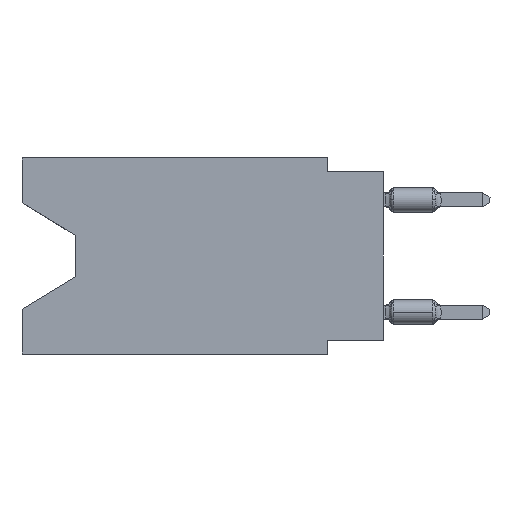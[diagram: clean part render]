
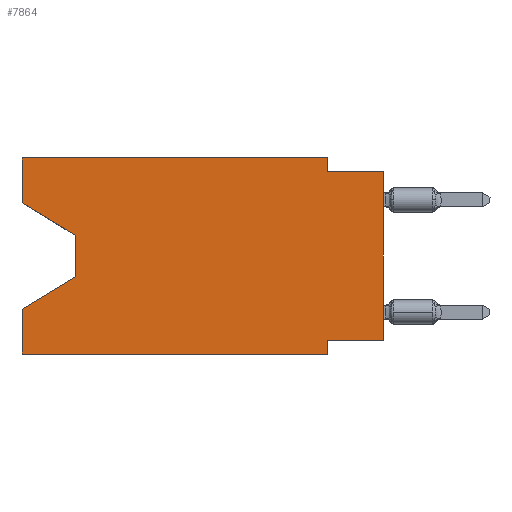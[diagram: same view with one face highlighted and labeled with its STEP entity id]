
A CAD part, left-side view. The second image highlights one B-rep face of the part: STEP entity #7864.
In plain terms, the highlighted planar face has unit normal (-1, 0, 0).
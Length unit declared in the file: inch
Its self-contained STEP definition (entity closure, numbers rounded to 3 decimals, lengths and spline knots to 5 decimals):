
#218 = ORIENTED_EDGE ( 'NONE', *, *, #9292, .T. ) ;
#283 = LINE ( 'NONE', #16107, #18698 ) ;
#565 = ORIENTED_EDGE ( 'NONE', *, *, #13233, .F. ) ;
#764 = CARTESIAN_POINT ( 'NONE',  ( 0., 0.645, -0.08025 ) ) ;
#988 = LINE ( 'NONE', #1072, #13239 ) ;
#1072 = CARTESIAN_POINT ( 'NONE',  ( 0., 0.645, 0. ) ) ;
#1233 = CARTESIAN_POINT ( 'NONE',  ( 0., 0., -0.325 ) ) ;
#1372 = EDGE_CURVE ( 'NONE', #12256, #6926, #4686, .T. ) ;
#1374 = VERTEX_POINT ( 'NONE', #11987 ) ;
#1750 = LINE ( 'NONE', #13599, #11968 ) ;
#2251 = VERTEX_POINT ( 'NONE', #5177 ) ;
#2436 = EDGE_CURVE ( 'NONE', #12759, #13123, #7107, .T. ) ;
#2453 = CARTESIAN_POINT ( 'NONE',  ( 0., 0.1, -0.35 ) ) ;
#2687 = EDGE_CURVE ( 'NONE', #2251, #11540, #3376, .T. ) ;
#3064 = ORIENTED_EDGE ( 'NONE', *, *, #10776, .F. ) ;
#3078 = ORIENTED_EDGE ( 'NONE', *, *, #2687, .F. ) ;
#3376 = LINE ( 'NONE', #6210, #5145 ) ;
#3420 = LINE ( 'NONE', #12143, #15102 ) ;
#3928 = CARTESIAN_POINT ( 'NONE',  ( 0., 0., -0.325 ) ) ;
#4103 = DIRECTION ( 'NONE',  ( 0., 0., 1. ) ) ;
#4405 = CARTESIAN_POINT ( 'NONE',  ( 0., 0.645, -0.08025 ) ) ;
#4410 = CARTESIAN_POINT ( 'NONE',  ( 0., 0.645, -0.35 ) ) ;
#4476 = LINE ( 'NONE', #10816, #8887 ) ;
#4483 = CARTESIAN_POINT ( 'NONE',  ( 0., 0.645, 0. ) ) ;
#4591 = DIRECTION ( 'NONE',  ( 0., 0., -1. ) ) ;
#4645 = DIRECTION ( 'NONE',  ( 0., 0., -1. ) ) ;
#4686 = LINE ( 'NONE', #4405, #13394 ) ;
#4913 = ORIENTED_EDGE ( 'NONE', *, *, #15853, .F. ) ;
#5021 = DIRECTION ( 'NONE',  ( 0., 0., -1. ) ) ;
#5068 = DIRECTION ( 'NONE',  ( 0., 0., 1. ) ) ;
#5093 = ORIENTED_EDGE ( 'NONE', *, *, #5103, .T. ) ;
#5103 = EDGE_CURVE ( 'NONE', #2251, #7350, #7436, .T. ) ;
#5145 = VECTOR ( 'NONE', #5068, 39.37008 ) ;
#5177 = CARTESIAN_POINT ( 'NONE',  ( 0., 0.645, -0.35 ) ) ;
#5553 = CARTESIAN_POINT ( 'NONE',  ( 0., 0.645, 0. ) ) ;
#5867 = ORIENTED_EDGE ( 'NONE', *, *, #6647, .F. ) ;
#6096 = CARTESIAN_POINT ( 'NONE',  ( 0., 0.645, 0. ) ) ;
#6210 = CARTESIAN_POINT ( 'NONE',  ( 0., 0.645, 0. ) ) ;
#6647 = EDGE_CURVE ( 'NONE', #10743, #1374, #15863, .T. ) ;
#6926 = VERTEX_POINT ( 'NONE', #7193 ) ;
#7012 = DIRECTION ( 'NONE',  ( 0., 1., 0. ) ) ;
#7064 = LINE ( 'NONE', #11426, #13480 ) ;
#7107 = LINE ( 'NONE', #1233, #17147 ) ;
#7193 = CARTESIAN_POINT ( 'NONE',  ( 0., 0.55, -0.138 ) ) ;
#7350 = VERTEX_POINT ( 'NONE', #2453 ) ;
#7428 = PLANE ( 'NONE',  #14197 ) ;
#7436 = LINE ( 'NONE', #4410, #8247 ) ;
#7521 = VECTOR ( 'NONE', #10127, 39.37008 ) ;
#7553 = CARTESIAN_POINT ( 'NONE',  ( 0., 0.55, -0.212 ) ) ;
#7864 = ADVANCED_FACE ( 'NONE', ( #16236 ), #7428, .F. ) ;
#8247 = VECTOR ( 'NONE', #13033, 39.37008 ) ;
#8756 = VERTEX_POINT ( 'NONE', #17181 ) ;
#8800 = CARTESIAN_POINT ( 'NONE',  ( 0., 0.645, -0.26975 ) ) ;
#8887 = VECTOR ( 'NONE', #5021, 39.37008 ) ;
#9042 = DIRECTION ( 'NONE',  ( 0., -0.855, -0.519 ) ) ;
#9056 = VERTEX_POINT ( 'NONE', #12149 ) ;
#9292 = EDGE_CURVE ( 'NONE', #6926, #10417, #283, .T. ) ;
#9681 = VECTOR ( 'NONE', #11416, 39.37008 ) ;
#10035 = LINE ( 'NONE', #17334, #7521 ) ;
#10127 = DIRECTION ( 'NONE',  ( 0., 0., 1. ) ) ;
#10173 = ORIENTED_EDGE ( 'NONE', *, *, #1372, .T. ) ;
#10417 = VERTEX_POINT ( 'NONE', #7553 ) ;
#10719 = ORIENTED_EDGE ( 'NONE', *, *, #2436, .F. ) ;
#10743 = VERTEX_POINT ( 'NONE', #5553 ) ;
#10776 = EDGE_CURVE ( 'NONE', #8756, #9056, #7064, .T. ) ;
#10816 = CARTESIAN_POINT ( 'NONE',  ( 0., 0.1, 0. ) ) ;
#10830 = EDGE_CURVE ( 'NONE', #10417, #11540, #1750, .T. ) ;
#11258 = EDGE_CURVE ( 'NONE', #1374, #8756, #4476, .T. ) ;
#11416 = DIRECTION ( 'NONE',  ( 0., -1., 0. ) ) ;
#11426 = CARTESIAN_POINT ( 'NONE',  ( 0., 0., -0.025 ) ) ;
#11540 = VERTEX_POINT ( 'NONE', #8800 ) ;
#11968 = VECTOR ( 'NONE', #17577, 39.37008 ) ;
#11987 = CARTESIAN_POINT ( 'NONE',  ( 0., 0.1, 0. ) ) ;
#12143 = CARTESIAN_POINT ( 'NONE',  ( 0., 0.1, -0.35 ) ) ;
#12149 = CARTESIAN_POINT ( 'NONE',  ( 0., 0., -0.025 ) ) ;
#12256 = VERTEX_POINT ( 'NONE', #764 ) ;
#12720 = ORIENTED_EDGE ( 'NONE', *, *, #14883, .T. ) ;
#12759 = VERTEX_POINT ( 'NONE', #3928 ) ;
#13033 = DIRECTION ( 'NONE',  ( 0., -1., 0. ) ) ;
#13123 = VERTEX_POINT ( 'NONE', #14909 ) ;
#13233 = EDGE_CURVE ( 'NONE', #12256, #10743, #988, .T. ) ;
#13239 = VECTOR ( 'NONE', #4103, 39.37008 ) ;
#13394 = VECTOR ( 'NONE', #9042, 39.37008 ) ;
#13480 = VECTOR ( 'NONE', #14166, 39.37008 ) ;
#13599 = CARTESIAN_POINT ( 'NONE',  ( 0., 0.55, -0.212 ) ) ;
#14166 = DIRECTION ( 'NONE',  ( 0., -1., 0. ) ) ;
#14197 = AXIS2_PLACEMENT_3D ( 'NONE', #6096, #14344, #4591 ) ;
#14344 = DIRECTION ( 'NONE',  ( 1., 0., 0. ) ) ;
#14701 = ORIENTED_EDGE ( 'NONE', *, *, #11258, .F. ) ;
#14883 = EDGE_CURVE ( 'NONE', #12759, #9056, #10035, .T. ) ;
#14909 = CARTESIAN_POINT ( 'NONE',  ( 0., 0.1, -0.325 ) ) ;
#15102 = VECTOR ( 'NONE', #17912, 39.37008 ) ;
#15853 = EDGE_CURVE ( 'NONE', #13123, #7350, #3420, .T. ) ;
#15863 = LINE ( 'NONE', #4483, #9681 ) ;
#16107 = CARTESIAN_POINT ( 'NONE',  ( 0., 0.55, -0.138 ) ) ;
#16236 = FACE_OUTER_BOUND ( 'NONE', #17703, .T. ) ;
#17147 = VECTOR ( 'NONE', #7012, 39.37008 ) ;
#17181 = CARTESIAN_POINT ( 'NONE',  ( 0., 0.1, -0.025 ) ) ;
#17334 = CARTESIAN_POINT ( 'NONE',  ( 0., 0., 0. ) ) ;
#17577 = DIRECTION ( 'NONE',  ( 0., 0.855, -0.519 ) ) ;
#17701 = ORIENTED_EDGE ( 'NONE', *, *, #10830, .T. ) ;
#17703 = EDGE_LOOP ( 'NONE', ( #10173, #218, #17701, #3078, #5093, #4913, #10719, #12720, #3064, #14701, #5867, #565 ) ) ;
#17912 = DIRECTION ( 'NONE',  ( 0., 0., -1. ) ) ;
#18698 = VECTOR ( 'NONE', #4645, 39.37008 ) ;
